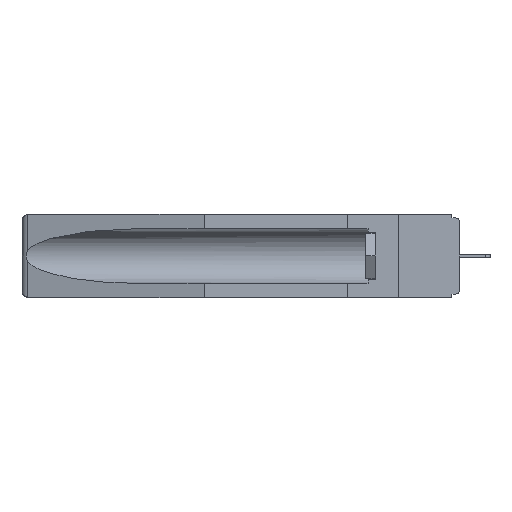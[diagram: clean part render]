
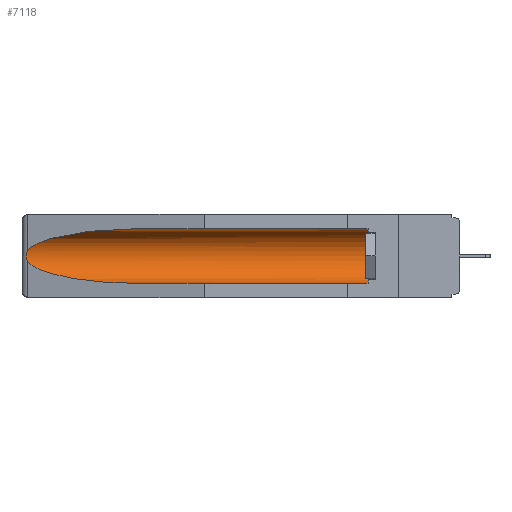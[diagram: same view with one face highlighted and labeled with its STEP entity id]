
A CAD part, left-side view. The second image highlights one B-rep face of the part: STEP entity #7118.
In plain terms, the highlighted cylindrical face has radius 2.857 mm (diameter 5.715 mm), a partial arc.
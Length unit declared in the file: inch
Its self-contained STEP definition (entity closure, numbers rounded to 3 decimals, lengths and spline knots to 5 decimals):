
#542 = EDGE_CURVE ( 'NONE', #22353, #14965, #4966, .T. ) ;
#740 = DIRECTION ( 'NONE',  ( 0., 1., 0. ) ) ;
#995 = ORIENTED_EDGE ( 'NONE', *, *, #542, .T. ) ;
#1438 = EDGE_CURVE ( 'NONE', #14965, #13458, #3064, .T. ) ;
#1808 = CIRCLE ( 'NONE', #17139, 0.1125 ) ;
#2015 = EDGE_CURVE ( 'NONE', #9418, #5676, #5631, .T. ) ;
#2705 = VERTEX_POINT ( 'NONE', #22418 ) ;
#3064 =( BOUNDED_CURVE ( )  B_SPLINE_CURVE ( 3, ( #13617, #14430, #13463, #11277 ),
 .UNSPECIFIED., .F., .T. ) 
 B_SPLINE_CURVE_WITH_KNOTS ( ( 4, 4 ),
 ( 4.71239, 6.08839 ),
 .UNSPECIFIED. ) 
 CURVE ( )  GEOMETRIC_REPRESENTATION_ITEM ( )  RATIONAL_B_SPLINE_CURVE ( ( 1., 0.848, 0.848, 1. ) ) 
 REPRESENTATION_ITEM ( '' )  );
#3489 = CARTESIAN_POINT ( 'NONE',  ( 0.26537, 1.52718, -0.14972 ) ) ;
#4405 = VECTOR ( 'NONE', #740, 39.37008 ) ;
#4619 = EDGE_CURVE ( 'NONE', #2705, #5676, #14379, .T. ) ;
#4783 = AXIS2_PLACEMENT_3D ( 'NONE', #17416, #8571, #15645 ) ;
#4937 = VECTOR ( 'NONE', #14655, 39.37008 ) ;
#4966 = LINE ( 'NONE', #22581, #4405 ) ;
#5386 = CARTESIAN_POINT ( 'NONE',  ( 0.2673, 1.5327, -0.16383 ) ) ;
#5631 =( BOUNDED_CURVE ( )  B_SPLINE_CURVE ( 3, ( #9229, #11347, #11995, #21420 ),
 .UNSPECIFIED., .F., .T. ) 
 B_SPLINE_CURVE_WITH_KNOTS ( ( 4, 4 ),
 ( 0.1948, 1.5708 ),
 .UNSPECIFIED. ) 
 CURVE ( )  GEOMETRIC_REPRESENTATION_ITEM ( )  RATIONAL_B_SPLINE_CURVE ( ( 1., 0.848, 0.848, 1. ) ) 
 REPRESENTATION_ITEM ( '' )  );
#5676 = VERTEX_POINT ( 'NONE', #12220 ) ;
#6840 = EDGE_LOOP ( 'NONE', ( #20840, #13369, #16004, #16721, #19353, #995 ) ) ;
#7118 = ADVANCED_FACE ( 'NONE', ( #22020 ), #12040, .F. ) ;
#7173 = CARTESIAN_POINT ( 'NONE',  ( 0.2675, 1.53308, -0.17534 ) ) ;
#7246 = CARTESIAN_POINT ( 'NONE',  ( 0.155, 0.126, -0.1715 ) ) ;
#8571 = DIRECTION ( 'NONE',  ( 0., 1., 0. ) ) ;
#8700 = CARTESIAN_POINT ( 'NONE',  ( 0.155, 1.07973, -0.059 ) ) ;
#9013 = CARTESIAN_POINT ( 'NONE',  ( 0.26655, 1.53094, -0.18657 ) ) ;
#9075 = DIRECTION ( 'NONE',  ( 0., 0., 1. ) ) ;
#9105 = B_SPLINE_CURVE_WITH_KNOTS ( 'NONE', 3,
 ( #3489, #19488, #15997, #5386, #17783, #7173, #19558, #9013, #21350, #10762 ),
 .UNSPECIFIED., .F., .F.,
 ( 4, 2, 2, 2, 4 ),
 ( 0., 0.00029, 0.00058, 0.00087, 0.00117 ),
 .UNSPECIFIED. ) ;
#9229 = CARTESIAN_POINT ( 'NONE',  ( 0.26537, 1.52718, -0.19328 ) ) ;
#9418 = VERTEX_POINT ( 'NONE', #20443 ) ;
#9933 = CARTESIAN_POINT ( 'NONE',  ( 0.26537, 1.52718, -0.14972 ) ) ;
#10762 = CARTESIAN_POINT ( 'NONE',  ( 0.26537, 1.52718, -0.19328 ) ) ;
#11203 = CARTESIAN_POINT ( 'NONE',  ( 0.155, -0.30754, -0.284 ) ) ;
#11277 = CARTESIAN_POINT ( 'NONE',  ( 0.26537, 1.52718, -0.14972 ) ) ;
#11347 = CARTESIAN_POINT ( 'NONE',  ( 0.25451, 1.48313, -0.24835 ) ) ;
#11995 = CARTESIAN_POINT ( 'NONE',  ( 0.21114, 1.30732, -0.284 ) ) ;
#12040 = CYLINDRICAL_SURFACE ( 'NONE', #4783, 0.1125 ) ;
#12220 = CARTESIAN_POINT ( 'NONE',  ( 0.155, 1.07973, -0.284 ) ) ;
#13369 = ORIENTED_EDGE ( 'NONE', *, *, #21723, .T. ) ;
#13458 = VERTEX_POINT ( 'NONE', #9933 ) ;
#13463 = CARTESIAN_POINT ( 'NONE',  ( 0.25451, 1.48313, -0.09465 ) ) ;
#13617 = CARTESIAN_POINT ( 'NONE',  ( 0.155, 1.07973, -0.059 ) ) ;
#14379 = LINE ( 'NONE', #11203, #4937 ) ;
#14430 = CARTESIAN_POINT ( 'NONE',  ( 0.21114, 1.30732, -0.059 ) ) ;
#14655 = DIRECTION ( 'NONE',  ( 0., 1., 0. ) ) ;
#14965 = VERTEX_POINT ( 'NONE', #8700 ) ;
#15645 = DIRECTION ( 'NONE',  ( 0., 0., 1. ) ) ;
#15997 = CARTESIAN_POINT ( 'NONE',  ( 0.26654, 1.53092, -0.15636 ) ) ;
#16004 = ORIENTED_EDGE ( 'NONE', *, *, #2015, .T. ) ;
#16721 = ORIENTED_EDGE ( 'NONE', *, *, #4619, .F. ) ;
#17139 = AXIS2_PLACEMENT_3D ( 'NONE', #7246, #19625, #9075 ) ;
#17254 = EDGE_CURVE ( 'NONE', #2705, #22353, #1808, .T. ) ;
#17416 = CARTESIAN_POINT ( 'NONE',  ( 0.155, -0.30754, -0.1715 ) ) ;
#17783 = CARTESIAN_POINT ( 'NONE',  ( 0.2675, 1.53308, -0.16763 ) ) ;
#19353 = ORIENTED_EDGE ( 'NONE', *, *, #17254, .T. ) ;
#19488 = CARTESIAN_POINT ( 'NONE',  ( 0.26597, 1.52961, -0.15275 ) ) ;
#19558 = CARTESIAN_POINT ( 'NONE',  ( 0.2673, 1.53269, -0.17917 ) ) ;
#19625 = DIRECTION ( 'NONE',  ( 0., -1., 0. ) ) ;
#20443 = CARTESIAN_POINT ( 'NONE',  ( 0.26537, 1.52718, -0.19328 ) ) ;
#20840 = ORIENTED_EDGE ( 'NONE', *, *, #1438, .T. ) ;
#21321 = CARTESIAN_POINT ( 'NONE',  ( 0.155, 0.126, -0.059 ) ) ;
#21350 = CARTESIAN_POINT ( 'NONE',  ( 0.26597, 1.5296, -0.19026 ) ) ;
#21420 = CARTESIAN_POINT ( 'NONE',  ( 0.155, 1.07973, -0.284 ) ) ;
#21723 = EDGE_CURVE ( 'NONE', #13458, #9418, #9105, .T. ) ;
#22020 = FACE_OUTER_BOUND ( 'NONE', #6840, .T. ) ;
#22353 = VERTEX_POINT ( 'NONE', #21321 ) ;
#22418 = CARTESIAN_POINT ( 'NONE',  ( 0.155, 0.126, -0.284 ) ) ;
#22581 = CARTESIAN_POINT ( 'NONE',  ( 0.155, -0.30754, -0.059 ) ) ;
